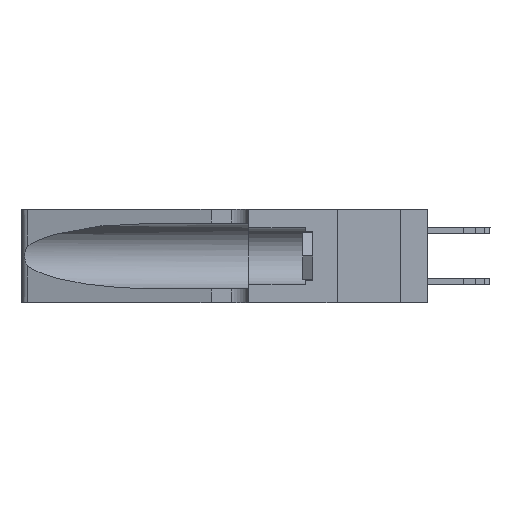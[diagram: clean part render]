
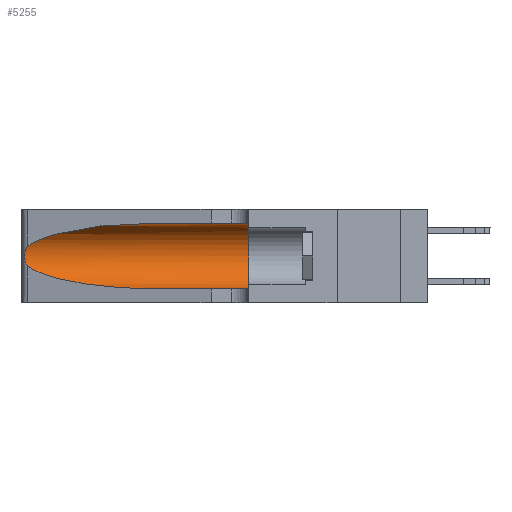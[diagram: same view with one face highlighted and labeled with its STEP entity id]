
A CAD part, left-side view. The second image highlights one B-rep face of the part: STEP entity #5255.
In plain terms, the highlighted cylindrical face has radius 3.308 mm (diameter 6.617 mm), a partial arc.
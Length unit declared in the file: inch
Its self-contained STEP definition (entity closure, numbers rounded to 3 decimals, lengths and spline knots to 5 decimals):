
#15 =( BOUNDED_CURVE ( )  B_SPLINE_CURVE ( 3, ( #4786, #6268, #17979, #9187 ),
 .UNSPECIFIED., .F., .F. ) 
 B_SPLINE_CURVE_WITH_KNOTS ( ( 4, 4 ),
 ( 3.44316, 4.71239 ),
 .UNSPECIFIED. ) 
 CURVE ( )  GEOMETRIC_REPRESENTATION_ITEM ( )  RATIONAL_B_SPLINE_CURVE ( ( 1., 0.87, 0.87, 1. ) ) 
 REPRESENTATION_ITEM ( '' )  );
#608 = CARTESIAN_POINT ( 'NONE',  ( 0.1305, 1.61858, 0.185 ) ) ;
#786 = CARTESIAN_POINT ( 'NONE',  ( 0.25487, 1.22718, 0.14631 ) ) ;
#1269 = EDGE_CURVE ( 'NONE', #12379, #11181, #15, .T. ) ;
#1494 = VERTEX_POINT ( 'NONE', #11426 ) ;
#1815 = CARTESIAN_POINT ( 'NONE',  ( 0.1305, 1.61858, 0.05475 ) ) ;
#1899 = CIRCLE ( 'NONE', #2528, 0.13025 ) ;
#2128 = DIRECTION ( 'NONE',  ( 0., 0., -1. ) ) ;
#2528 = AXIS2_PLACEMENT_3D ( 'NONE', #3288, #6282, #13610 ) ;
#3288 = CARTESIAN_POINT ( 'NONE',  ( 0.1305, 0.35, 0.185 ) ) ;
#3361 = VERTEX_POINT ( 'NONE', #17422 ) ;
#3537 = CARTESIAN_POINT ( 'NONE',  ( 0.25487, 1.22718, 0.14631 ) ) ;
#3725 = CARTESIAN_POINT ( 'NONE',  ( 0.25854, 1.2359, 0.20912 ) ) ;
#3919 = LINE ( 'NONE', #6863, #17423 ) ;
#4296 = CARTESIAN_POINT ( 'NONE',  ( 0.1305, 0.72297, 0.31525 ) ) ;
#4543 = EDGE_CURVE ( 'NONE', #11181, #16589, #18833, .T. ) ;
#4743 = ORIENTED_EDGE ( 'NONE', *, *, #10517, .F. ) ;
#4786 = CARTESIAN_POINT ( 'NONE',  ( 0.25487, 1.22718, 0.14631 ) ) ;
#5255 = ADVANCED_FACE ( 'NONE', ( #12599 ), #9155, .F. ) ;
#6268 = CARTESIAN_POINT ( 'NONE',  ( 0.2373, 1.15595, 0.08982 ) ) ;
#6282 = DIRECTION ( 'NONE',  ( 0., 1., 0. ) ) ;
#6553 = CARTESIAN_POINT ( 'NONE',  ( 0.25639, 1.23184, 0.21858 ) ) ;
#6777 = EDGE_CURVE ( 'NONE', #10393, #3361, #8222, .T. ) ;
#6863 = CARTESIAN_POINT ( 'NONE',  ( 0.1305, 1.61858, 0.31525 ) ) ;
#6991 = CARTESIAN_POINT ( 'NONE',  ( 0.2373, 1.15595, 0.28018 ) ) ;
#7472 = CARTESIAN_POINT ( 'NONE',  ( 0.1305, 0.35, 0.05475 ) ) ;
#7545 = EDGE_CURVE ( 'NONE', #3361, #12379, #10757, .T. ) ;
#8222 =( BOUNDED_CURVE ( )  B_SPLINE_CURVE ( 3, ( #14929, #15592, #6991, #14533 ),
 .UNSPECIFIED., .F., .F. ) 
 B_SPLINE_CURVE_WITH_KNOTS ( ( 4, 4 ),
 ( 1.5708, 2.84003 ),
 .UNSPECIFIED. ) 
 CURVE ( )  GEOMETRIC_REPRESENTATION_ITEM ( )  RATIONAL_B_SPLINE_CURVE ( ( 1., 0.87, 0.87, 1. ) ) 
 REPRESENTATION_ITEM ( '' )  );
#8377 = EDGE_LOOP ( 'NONE', ( #15779, #11406, #14371, #9901, #15691, #4743 ) ) ;
#8747 = DIRECTION ( 'NONE',  ( 0., -1., 0. ) ) ;
#9082 = EDGE_CURVE ( 'NONE', #1494, #16589, #1899, .T. ) ;
#9155 = CYLINDRICAL_SURFACE ( 'NONE', #10905, 0.13025 ) ;
#9187 = CARTESIAN_POINT ( 'NONE',  ( 0.1305, 0.72297, 0.05475 ) ) ;
#9450 = CARTESIAN_POINT ( 'NONE',  ( 0.25555, 1.22994, 0.2215 ) ) ;
#9525 = CARTESIAN_POINT ( 'NONE',  ( 0.26017, 1.23833, 0.17102 ) ) ;
#9901 = ORIENTED_EDGE ( 'NONE', *, *, #4543, .T. ) ;
#10393 = VERTEX_POINT ( 'NONE', #4296 ) ;
#10517 = EDGE_CURVE ( 'NONE', #10393, #1494, #3919, .T. ) ;
#10757 = B_SPLINE_CURVE_WITH_KNOTS ( 'NONE', 3,
 ( #11128, #9450, #6553, #10994, #3725, #13928, #16911, #13874, #9525, #11064, #18446, #15549, #13805, #786 ),
 .UNSPECIFIED., .F., .F.,
 ( 4, 2, 2, 2, 2, 2, 4 ),
 ( 0., 0.00027, 0.00053, 0.00107, 0.0016, 0.00187, 0.00214 ),
 .UNSPECIFIED. ) ;
#10806 = DIRECTION ( 'NONE',  ( 0., -1., 0. ) ) ;
#10905 = AXIS2_PLACEMENT_3D ( 'NONE', #608, #10806, #2128 ) ;
#10994 = CARTESIAN_POINT ( 'NONE',  ( 0.25787, 1.23484, 0.2124 ) ) ;
#11064 = CARTESIAN_POINT ( 'NONE',  ( 0.25856, 1.23593, 0.16098 ) ) ;
#11128 = CARTESIAN_POINT ( 'NONE',  ( 0.25487, 1.22718, 0.22369 ) ) ;
#11181 = VERTEX_POINT ( 'NONE', #11616 ) ;
#11406 = ORIENTED_EDGE ( 'NONE', *, *, #7545, .T. ) ;
#11426 = CARTESIAN_POINT ( 'NONE',  ( 0.1305, 0.35, 0.31525 ) ) ;
#11616 = CARTESIAN_POINT ( 'NONE',  ( 0.1305, 0.72297, 0.05475 ) ) ;
#12379 = VERTEX_POINT ( 'NONE', #3537 ) ;
#12599 = FACE_OUTER_BOUND ( 'NONE', #8377, .T. ) ;
#13495 = DIRECTION ( 'NONE',  ( 0., -1., 0. ) ) ;
#13610 = DIRECTION ( 'NONE',  ( 0., 0., 1. ) ) ;
#13805 = CARTESIAN_POINT ( 'NONE',  ( 0.25555, 1.22993, 0.14849 ) ) ;
#13874 = CARTESIAN_POINT ( 'NONE',  ( 0.26075, 1.23896, 0.178 ) ) ;
#13928 = CARTESIAN_POINT ( 'NONE',  ( 0.26018, 1.23835, 0.19895 ) ) ;
#14371 = ORIENTED_EDGE ( 'NONE', *, *, #1269, .T. ) ;
#14533 = CARTESIAN_POINT ( 'NONE',  ( 0.25487, 1.22718, 0.22369 ) ) ;
#14929 = CARTESIAN_POINT ( 'NONE',  ( 0.1305, 0.72297, 0.31525 ) ) ;
#15549 = CARTESIAN_POINT ( 'NONE',  ( 0.25639, 1.23186, 0.15144 ) ) ;
#15592 = CARTESIAN_POINT ( 'NONE',  ( 0.18966, 0.96281, 0.31525 ) ) ;
#15691 = ORIENTED_EDGE ( 'NONE', *, *, #9082, .F. ) ;
#15779 = ORIENTED_EDGE ( 'NONE', *, *, #6777, .T. ) ;
#16589 = VERTEX_POINT ( 'NONE', #7472 ) ;
#16911 = CARTESIAN_POINT ( 'NONE',  ( 0.26075, 1.23896, 0.19203 ) ) ;
#17422 = CARTESIAN_POINT ( 'NONE',  ( 0.25487, 1.22718, 0.22369 ) ) ;
#17423 = VECTOR ( 'NONE', #8747, 39.37008 ) ;
#17460 = VECTOR ( 'NONE', #13495, 39.37008 ) ;
#17979 = CARTESIAN_POINT ( 'NONE',  ( 0.18966, 0.96281, 0.05475 ) ) ;
#18446 = CARTESIAN_POINT ( 'NONE',  ( 0.25789, 1.23486, 0.15765 ) ) ;
#18833 = LINE ( 'NONE', #1815, #17460 ) ;
